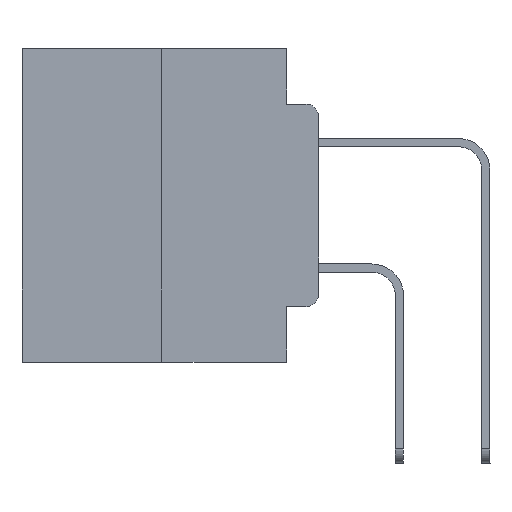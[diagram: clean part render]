
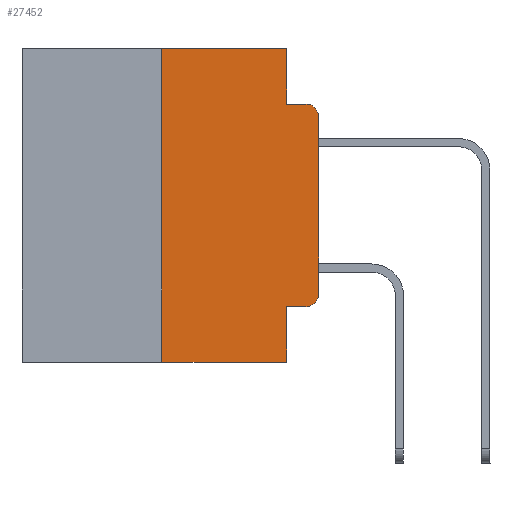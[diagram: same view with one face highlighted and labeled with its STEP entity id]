
A CAD part, left-side view. The second image highlights one B-rep face of the part: STEP entity #27452.
In plain terms, the highlighted planar face has unit normal (-1, 0, 0).
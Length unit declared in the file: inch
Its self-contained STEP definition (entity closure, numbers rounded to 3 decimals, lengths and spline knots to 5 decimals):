
#34 = LINE ( 'NONE', #13573, #22576 ) ;
#214 = DIRECTION ( 'NONE',  ( 0., -1., 0. ) ) ;
#860 = CARTESIAN_POINT ( 'NONE',  ( 0., 0.051, 0. ) ) ;
#1263 = ORIENTED_EDGE ( 'NONE', *, *, #21673, .T. ) ;
#1700 = VECTOR ( 'NONE', #10583, 39.37008 ) ;
#1802 = ORIENTED_EDGE ( 'NONE', *, *, #5499, .F. ) ;
#2085 = DIRECTION ( 'NONE',  ( 1., 0., 0. ) ) ;
#2087 = VECTOR ( 'NONE', #7863, 39.37008 ) ;
#3669 = EDGE_CURVE ( 'NONE', #25085, #8036, #15753, .T. ) ;
#3774 = VECTOR ( 'NONE', #214, 39.37008 ) ;
#4126 = ORIENTED_EDGE ( 'NONE', *, *, #24703, .F. ) ;
#4214 = DIRECTION ( 'NONE',  ( -1., 0., 0. ) ) ;
#4596 = DIRECTION ( 'NONE',  ( 0., 0., -1. ) ) ;
#4620 = ORIENTED_EDGE ( 'NONE', *, *, #18694, .T. ) ;
#4680 = VECTOR ( 'NONE', #11786, 39.37008 ) ;
#4791 = VERTEX_POINT ( 'NONE', #16351 ) ;
#5499 = EDGE_CURVE ( 'NONE', #24582, #4791, #20843, .T. ) ;
#5628 = CARTESIAN_POINT ( 'NONE',  ( 0., 0.473, 0. ) ) ;
#6025 = AXIS2_PLACEMENT_3D ( 'NONE', #25702, #12773, #27793 ) ;
#6912 = CARTESIAN_POINT ( 'NONE',  ( 0., 0., -0.1085 ) ) ;
#7546 = EDGE_CURVE ( 'NONE', #19984, #24582, #22153, .T. ) ;
#7863 = DIRECTION ( 'NONE',  ( 0., -1., 0. ) ) ;
#7934 = ORIENTED_EDGE ( 'NONE', *, *, #7546, .F. ) ;
#7998 = DIRECTION ( 'NONE',  ( 0., 0., 1. ) ) ;
#8036 = VERTEX_POINT ( 'NONE', #15580 ) ;
#9261 = VECTOR ( 'NONE', #7998, 39.37008 ) ;
#9456 = CIRCLE ( 'NONE', #6025, 0.02 ) ;
#9928 = LINE ( 'NONE', #17645, #26493 ) ;
#10416 = ORIENTED_EDGE ( 'NONE', *, *, #26627, .F. ) ;
#10583 = DIRECTION ( 'NONE',  ( 0., 0., 1. ) ) ;
#10632 = CARTESIAN_POINT ( 'NONE',  ( 0., 0.051, -0.4115 ) ) ;
#10904 = VERTEX_POINT ( 'NONE', #27790 ) ;
#11126 = CARTESIAN_POINT ( 'NONE',  ( 0., 0.051, -0.0885 ) ) ;
#11322 = CARTESIAN_POINT ( 'NONE',  ( 0., 0.25, -0.5 ) ) ;
#11786 = DIRECTION ( 'NONE',  ( 0., 0., -1. ) ) ;
#12678 = CARTESIAN_POINT ( 'NONE',  ( 0., 0., 0. ) ) ;
#12773 = DIRECTION ( 'NONE',  ( -1., 0., 0. ) ) ;
#13573 = CARTESIAN_POINT ( 'NONE',  ( 0., 0.473, -0.5 ) ) ;
#13636 = EDGE_CURVE ( 'NONE', #27871, #10904, #20367, .T. ) ;
#13805 = CARTESIAN_POINT ( 'NONE',  ( 0., 0.051, 0. ) ) ;
#15580 = CARTESIAN_POINT ( 'NONE',  ( 0., 0.25, 0. ) ) ;
#15753 = LINE ( 'NONE', #18896, #9261 ) ;
#16351 = CARTESIAN_POINT ( 'NONE',  ( 0., 0.02, -0.0885 ) ) ;
#16809 = DIRECTION ( 'NONE',  ( 0., -1., 0. ) ) ;
#17035 = VECTOR ( 'NONE', #16809, 39.37008 ) ;
#17294 = EDGE_CURVE ( 'NONE', #10904, #19330, #19179, .T. ) ;
#17330 = PLANE ( 'NONE',  #19159 ) ;
#17356 = CARTESIAN_POINT ( 'NONE',  ( 0., 0.02, -0.3915 ) ) ;
#17417 = DIRECTION ( 'NONE',  ( 0., 0., -1. ) ) ;
#17559 = CARTESIAN_POINT ( 'NONE',  ( 0., 0.051, -0.5 ) ) ;
#17645 = CARTESIAN_POINT ( 'NONE',  ( 0., 0.051, 0. ) ) ;
#18421 = EDGE_LOOP ( 'NONE', ( #26115, #1263, #1802, #7934, #4126, #19791, #4620, #10416, #19522, #20571 ) ) ;
#18437 = VERTEX_POINT ( 'NONE', #10632 ) ;
#18694 = EDGE_CURVE ( 'NONE', #25085, #24332, #34, .T. ) ;
#18896 = CARTESIAN_POINT ( 'NONE',  ( 0., 0.25, 0. ) ) ;
#19159 = AXIS2_PLACEMENT_3D ( 'NONE', #23850, #2085, #17417 ) ;
#19179 = LINE ( 'NONE', #12678, #1700 ) ;
#19330 = VERTEX_POINT ( 'NONE', #6912 ) ;
#19522 = ORIENTED_EDGE ( 'NONE', *, *, #20922, .T. ) ;
#19540 = DIRECTION ( 'NONE',  ( 0., 0., -1. ) ) ;
#19569 = LINE ( 'NONE', #5628, #2087 ) ;
#19791 = ORIENTED_EDGE ( 'NONE', *, *, #3669, .F. ) ;
#19984 = VERTEX_POINT ( 'NONE', #13805 ) ;
#20367 = CIRCLE ( 'NONE', #23267, 0.02 ) ;
#20571 = ORIENTED_EDGE ( 'NONE', *, *, #13636, .T. ) ;
#20843 = LINE ( 'NONE', #11126, #3774 ) ;
#20922 = EDGE_CURVE ( 'NONE', #18437, #27871, #22131, .T. ) ;
#20997 = CARTESIAN_POINT ( 'NONE',  ( 0., 0.02, -0.4115 ) ) ;
#21673 = EDGE_CURVE ( 'NONE', #19330, #4791, #9456, .T. ) ;
#22131 = LINE ( 'NONE', #25360, #17035 ) ;
#22153 = LINE ( 'NONE', #860, #4680 ) ;
#22160 = FACE_OUTER_BOUND ( 'NONE', #18421, .T. ) ;
#22576 = VECTOR ( 'NONE', #24266, 39.37008 ) ;
#22670 = CARTESIAN_POINT ( 'NONE',  ( 0., 0.051, -0.0885 ) ) ;
#23267 = AXIS2_PLACEMENT_3D ( 'NONE', #17356, #4214, #19540 ) ;
#23850 = CARTESIAN_POINT ( 'NONE',  ( 0., 0.473, 0. ) ) ;
#24266 = DIRECTION ( 'NONE',  ( 0., -1., 0. ) ) ;
#24332 = VERTEX_POINT ( 'NONE', #17559 ) ;
#24582 = VERTEX_POINT ( 'NONE', #22670 ) ;
#24703 = EDGE_CURVE ( 'NONE', #8036, #19984, #19569, .T. ) ;
#25085 = VERTEX_POINT ( 'NONE', #11322 ) ;
#25360 = CARTESIAN_POINT ( 'NONE',  ( 0., 0.051, -0.4115 ) ) ;
#25702 = CARTESIAN_POINT ( 'NONE',  ( 0., 0.02, -0.1085 ) ) ;
#26115 = ORIENTED_EDGE ( 'NONE', *, *, #17294, .T. ) ;
#26493 = VECTOR ( 'NONE', #4596, 39.37008 ) ;
#26627 = EDGE_CURVE ( 'NONE', #18437, #24332, #9928, .T. ) ;
#27452 = ADVANCED_FACE ( 'NONE', ( #22160 ), #17330, .F. ) ;
#27790 = CARTESIAN_POINT ( 'NONE',  ( 0., 0., -0.3915 ) ) ;
#27793 = DIRECTION ( 'NONE',  ( 0., 0., -1. ) ) ;
#27871 = VERTEX_POINT ( 'NONE', #20997 ) ;
